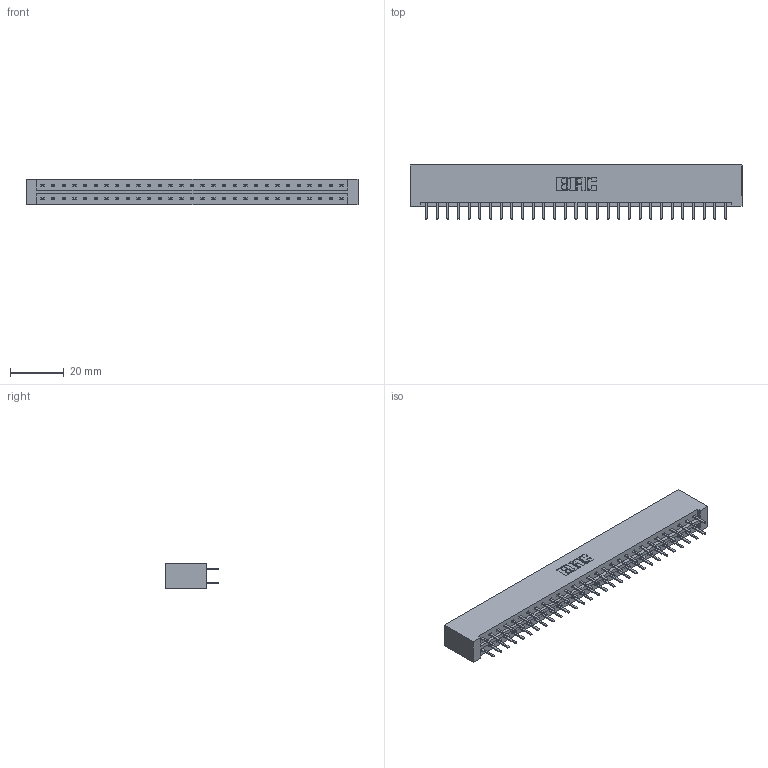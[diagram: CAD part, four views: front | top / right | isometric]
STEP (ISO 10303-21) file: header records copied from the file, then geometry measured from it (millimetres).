
FILE_DESCRIPTION (( 'STEP AP203' ), '1' );
FILE_NAME ('833-058-520-201.STEP', '2020-06-04T23:55:10', ( '' ), ( '' ), 'SwSTEP 2.0', 'SolidWorks 2020', '' );
FILE_SCHEMA (( 'CONFIG_CONTROL_DESIGN' ));
Length unit declared in the file: inch
Products named in the file (3): 345-292-001_345-293-120; 833 Part_Lugless; 833-058-520-201
Assembly tree (59 placements, depth 2):
  833-058-520-201
    833 Part_Lugless
    345-292-001_345-293-120  x58
Bounding box: 123.16 x 20.02 x 9.4 mm (x, y, z)
Volume: 13059.6 mm3; surface area: 15256.8 mm2
Topology: 59 solids, 59 shells, 3354 faces, 9741 edges, 6338 vertices
Faces by surface type: plane 2270, cylinder 1084
Entity records: 20175 total; most frequent: CARTESIAN_POINT 3370, ORIENTED_EDGE 3294, DIRECTION 2883, EDGE_CURVE 1647, VECTOR 1523, LINE 1523, VERTEX_POINT 1094, AXIS2_PLACEMENT_3D 680
